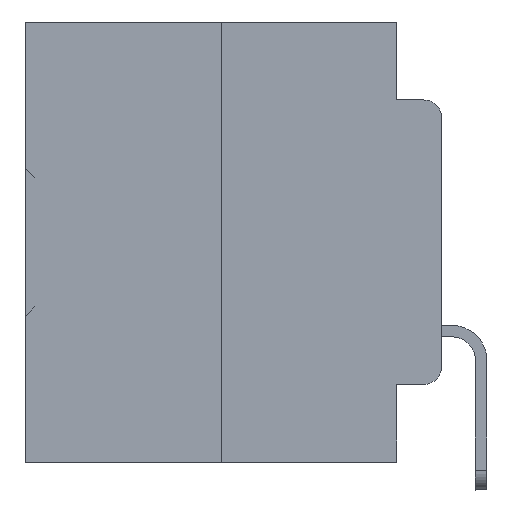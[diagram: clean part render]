
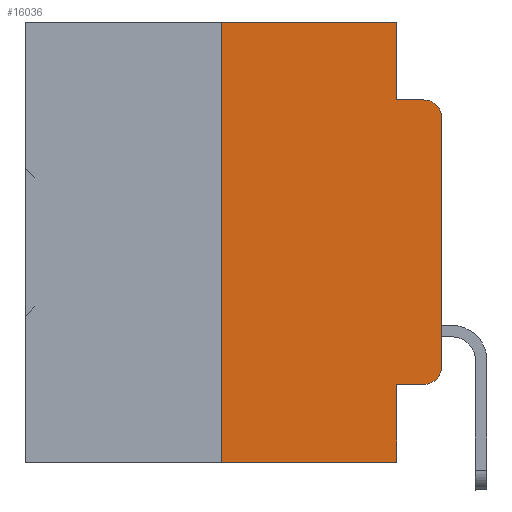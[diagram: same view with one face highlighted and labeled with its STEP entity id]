
A CAD part, left-side view. The second image highlights one B-rep face of the part: STEP entity #16036.
In plain terms, the highlighted planar face has unit normal (-1, 0, 0).
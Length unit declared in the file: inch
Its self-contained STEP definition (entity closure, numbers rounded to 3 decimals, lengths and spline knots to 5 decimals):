
#243 = EDGE_CURVE ( 'NONE', #35296, #427, #32079, .T. ) ;
#427 = VERTEX_POINT ( 'NONE', #1049 ) ;
#848 = PLANE ( 'NONE',  #33599 ) ;
#1036 = DIRECTION ( 'NONE',  ( 0., 0., -1. ) ) ;
#1049 = CARTESIAN_POINT ( 'NONE',  ( 0., 0.051, -0.5 ) ) ;
#1466 = VERTEX_POINT ( 'NONE', #37580 ) ;
#2315 = VERTEX_POINT ( 'NONE', #37442 ) ;
#2696 = VECTOR ( 'NONE', #6307, 39.37008 ) ;
#3391 = CARTESIAN_POINT ( 'NONE',  ( 0., 0.473, 0. ) ) ;
#5299 = VERTEX_POINT ( 'NONE', #24126 ) ;
#5431 = CARTESIAN_POINT ( 'NONE',  ( 0., 0., 0. ) ) ;
#6307 = DIRECTION ( 'NONE',  ( 0., -1., 0. ) ) ;
#7535 = LINE ( 'NONE', #22626, #27337 ) ;
#7537 = DIRECTION ( 'NONE',  ( 0., 0., -1. ) ) ;
#7672 = EDGE_CURVE ( 'NONE', #35296, #2315, #7535, .T. ) ;
#8224 = EDGE_CURVE ( 'NONE', #26800, #21594, #23348, .T. ) ;
#8811 = DIRECTION ( 'NONE',  ( 0., 0., 1. ) ) ;
#8830 = EDGE_LOOP ( 'NONE', ( #26241, #35757, #25882, #21934, #18953, #16085, #23211, #13436, #9072, #21840 ) ) ;
#8902 = DIRECTION ( 'NONE',  ( 0., 0., 1. ) ) ;
#8968 = EDGE_CURVE ( 'NONE', #21716, #34142, #33954, .T. ) ;
#9059 = VECTOR ( 'NONE', #10562, 39.37008 ) ;
#9072 = ORIENTED_EDGE ( 'NONE', *, *, #7672, .T. ) ;
#10562 = DIRECTION ( 'NONE',  ( 0., -1., 0. ) ) ;
#11248 = DIRECTION ( 'NONE',  ( 0., 0., -1. ) ) ;
#11744 = CARTESIAN_POINT ( 'NONE',  ( 0., 0.051, 0. ) ) ;
#11787 = LINE ( 'NONE', #20522, #25170 ) ;
#11870 = CARTESIAN_POINT ( 'NONE',  ( 0., 0.051, -0.4115 ) ) ;
#13436 = ORIENTED_EDGE ( 'NONE', *, *, #243, .F. ) ;
#14545 = CARTESIAN_POINT ( 'NONE',  ( 0., 0.02, -0.3915 ) ) ;
#14603 = CARTESIAN_POINT ( 'NONE',  ( 0., 0.02, -0.1085 ) ) ;
#15610 = VECTOR ( 'NONE', #8811, 39.37008 ) ;
#15810 = EDGE_CURVE ( 'NONE', #29568, #5299, #18091, .T. ) ;
#16036 = ADVANCED_FACE ( 'NONE', ( #27402 ), #848, .F. ) ;
#16085 = ORIENTED_EDGE ( 'NONE', *, *, #8224, .F. ) ;
#16349 = VECTOR ( 'NONE', #8902, 39.37008 ) ;
#17247 = DIRECTION ( 'NONE',  ( 0., -1., 0. ) ) ;
#17905 = DIRECTION ( 'NONE',  ( 0., 0., -1. ) ) ;
#18091 = CIRCLE ( 'NONE', #34816, 0.02 ) ;
#18887 = EDGE_CURVE ( 'NONE', #21594, #21716, #21400, .T. ) ;
#18953 = ORIENTED_EDGE ( 'NONE', *, *, #18887, .F. ) ;
#19183 = EDGE_CURVE ( 'NONE', #1466, #29568, #37800, .T. ) ;
#19291 = VECTOR ( 'NONE', #37062, 39.37008 ) ;
#20435 = CARTESIAN_POINT ( 'NONE',  ( 0., 0.25, 0. ) ) ;
#20522 = CARTESIAN_POINT ( 'NONE',  ( 0., 0.473, -0.5 ) ) ;
#20759 = CARTESIAN_POINT ( 'NONE',  ( 0., 0.051, -0.0885 ) ) ;
#20802 = DIRECTION ( 'NONE',  ( -1., 0., 0. ) ) ;
#21400 = LINE ( 'NONE', #3391, #2696 ) ;
#21574 = CARTESIAN_POINT ( 'NONE',  ( 0., 0.473, 0. ) ) ;
#21594 = VERTEX_POINT ( 'NONE', #33938 ) ;
#21716 = VERTEX_POINT ( 'NONE', #11744 ) ;
#21840 = ORIENTED_EDGE ( 'NONE', *, *, #31612, .T. ) ;
#21853 = EDGE_CURVE ( 'NONE', #34142, #5299, #27462, .T. ) ;
#21934 = ORIENTED_EDGE ( 'NONE', *, *, #8968, .F. ) ;
#22626 = CARTESIAN_POINT ( 'NONE',  ( 0., 0.051, -0.4115 ) ) ;
#22682 = CARTESIAN_POINT ( 'NONE',  ( 0., 0.051, 0. ) ) ;
#22920 = EDGE_CURVE ( 'NONE', #26800, #427, #11787, .T. ) ;
#23211 = ORIENTED_EDGE ( 'NONE', *, *, #22920, .T. ) ;
#23348 = LINE ( 'NONE', #20435, #15610 ) ;
#23462 = DIRECTION ( 'NONE',  ( -1., 0., 0. ) ) ;
#24126 = CARTESIAN_POINT ( 'NONE',  ( 0., 0.02, -0.0885 ) ) ;
#25119 = CARTESIAN_POINT ( 'NONE',  ( 0., 0.051, -0.0885 ) ) ;
#25170 = VECTOR ( 'NONE', #17247, 39.37008 ) ;
#25882 = ORIENTED_EDGE ( 'NONE', *, *, #21853, .F. ) ;
#26241 = ORIENTED_EDGE ( 'NONE', *, *, #19183, .T. ) ;
#26800 = VERTEX_POINT ( 'NONE', #30630 ) ;
#27337 = VECTOR ( 'NONE', #37190, 39.37008 ) ;
#27402 = FACE_OUTER_BOUND ( 'NONE', #8830, .T. ) ;
#27462 = LINE ( 'NONE', #25119, #9059 ) ;
#27592 = DIRECTION ( 'NONE',  ( 1., 0., 0. ) ) ;
#29568 = VERTEX_POINT ( 'NONE', #34122 ) ;
#30630 = CARTESIAN_POINT ( 'NONE',  ( 0., 0.25, -0.5 ) ) ;
#31612 = EDGE_CURVE ( 'NONE', #2315, #1466, #33975, .T. ) ;
#32079 = LINE ( 'NONE', #34090, #36559 ) ;
#33599 = AXIS2_PLACEMENT_3D ( 'NONE', #21574, #27592, #1036 ) ;
#33938 = CARTESIAN_POINT ( 'NONE',  ( 0., 0.25, 0. ) ) ;
#33954 = LINE ( 'NONE', #22682, #19291 ) ;
#33975 = CIRCLE ( 'NONE', #37086, 0.02 ) ;
#34090 = CARTESIAN_POINT ( 'NONE',  ( 0., 0.051, 0. ) ) ;
#34122 = CARTESIAN_POINT ( 'NONE',  ( 0., 0., -0.1085 ) ) ;
#34142 = VERTEX_POINT ( 'NONE', #20759 ) ;
#34816 = AXIS2_PLACEMENT_3D ( 'NONE', #14603, #20802, #17905 ) ;
#35296 = VERTEX_POINT ( 'NONE', #11870 ) ;
#35757 = ORIENTED_EDGE ( 'NONE', *, *, #15810, .T. ) ;
#36559 = VECTOR ( 'NONE', #7537, 39.37008 ) ;
#37062 = DIRECTION ( 'NONE',  ( 0., 0., -1. ) ) ;
#37086 = AXIS2_PLACEMENT_3D ( 'NONE', #14545, #23462, #11248 ) ;
#37190 = DIRECTION ( 'NONE',  ( 0., -1., 0. ) ) ;
#37442 = CARTESIAN_POINT ( 'NONE',  ( 0., 0.02, -0.4115 ) ) ;
#37580 = CARTESIAN_POINT ( 'NONE',  ( 0., 0., -0.3915 ) ) ;
#37800 = LINE ( 'NONE', #5431, #16349 ) ;
